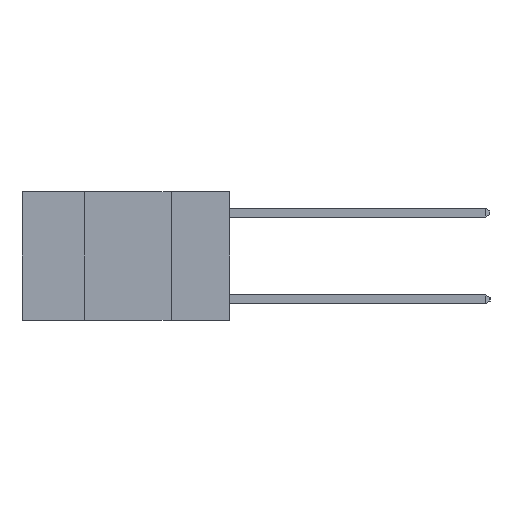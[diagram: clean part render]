
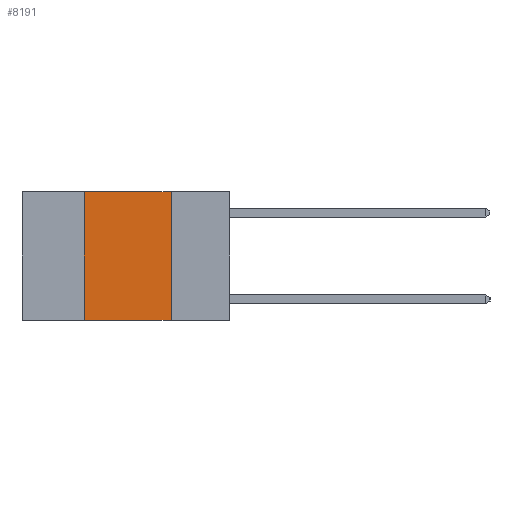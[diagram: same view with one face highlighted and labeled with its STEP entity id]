
A CAD part, left-side view. The second image highlights one B-rep face of the part: STEP entity #8191.
In plain terms, the highlighted planar face has unit normal (-1, 0, 0).
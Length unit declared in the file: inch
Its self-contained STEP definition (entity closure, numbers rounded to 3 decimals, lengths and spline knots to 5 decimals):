
#78 = CARTESIAN_POINT ( 'NONE',  ( 0., 0.42, 0. ) ) ;
#105 = ORIENTED_EDGE ( 'NONE', *, *, #7610, .F. ) ;
#230 = ORIENTED_EDGE ( 'NONE', *, *, #1454, .F. ) ;
#549 = CARTESIAN_POINT ( 'NONE',  ( 0., 0.17, -0.37 ) ) ;
#808 = VECTOR ( 'NONE', #7564, 39.37008 ) ;
#1454 = EDGE_CURVE ( 'NONE', #3037, #4385, #11405, .T. ) ;
#1978 = LINE ( 'NONE', #10693, #6566 ) ;
#1998 = EDGE_CURVE ( 'NONE', #4385, #9702, #5747, .T. ) ;
#2084 = CARTESIAN_POINT ( 'NONE',  ( 0., 0.6, 0. ) ) ;
#2086 = EDGE_CURVE ( 'NONE', #3037, #3465, #9427, .T. ) ;
#2439 = PLANE ( 'NONE',  #2926 ) ;
#2926 = AXIS2_PLACEMENT_3D ( 'NONE', #4290, #10646, #5195 ) ;
#3037 = VERTEX_POINT ( 'NONE', #10985 ) ;
#3465 = VERTEX_POINT ( 'NONE', #549 ) ;
#4176 = VECTOR ( 'NONE', #5009, 39.37008 ) ;
#4290 = CARTESIAN_POINT ( 'NONE',  ( 0., 0.6, 0. ) ) ;
#4385 = VERTEX_POINT ( 'NONE', #78 ) ;
#4529 = EDGE_LOOP ( 'NONE', ( #105, #7155, #230, #6249 ) ) ;
#5009 = DIRECTION ( 'NONE',  ( 0., 0., 1. ) ) ;
#5195 = DIRECTION ( 'NONE',  ( 0., 0., -1. ) ) ;
#5747 = LINE ( 'NONE', #2084, #808 ) ;
#6169 = DIRECTION ( 'NONE',  ( 0., 0., -1. ) ) ;
#6249 = ORIENTED_EDGE ( 'NONE', *, *, #2086, .T. ) ;
#6566 = VECTOR ( 'NONE', #6169, 39.37008 ) ;
#6991 = VECTOR ( 'NONE', #9535, 39.37008 ) ;
#7155 = ORIENTED_EDGE ( 'NONE', *, *, #1998, .F. ) ;
#7503 = CARTESIAN_POINT ( 'NONE',  ( 0., 0.17, 0. ) ) ;
#7564 = DIRECTION ( 'NONE',  ( 0., -1., 0. ) ) ;
#7610 = EDGE_CURVE ( 'NONE', #9702, #3465, #1978, .T. ) ;
#8191 = ADVANCED_FACE ( 'NONE', ( #8566 ), #2439, .F. ) ;
#8566 = FACE_OUTER_BOUND ( 'NONE', #4529, .T. ) ;
#8625 = CARTESIAN_POINT ( 'NONE',  ( 0., 0.6, -0.37 ) ) ;
#9427 = LINE ( 'NONE', #8625, #6991 ) ;
#9535 = DIRECTION ( 'NONE',  ( 0., -1., 0. ) ) ;
#9548 = CARTESIAN_POINT ( 'NONE',  ( 0., 0.42, 0. ) ) ;
#9702 = VERTEX_POINT ( 'NONE', #7503 ) ;
#10646 = DIRECTION ( 'NONE',  ( 1., 0., 0. ) ) ;
#10693 = CARTESIAN_POINT ( 'NONE',  ( 0., 0.17, 0. ) ) ;
#10985 = CARTESIAN_POINT ( 'NONE',  ( 0., 0.42, -0.37 ) ) ;
#11405 = LINE ( 'NONE', #9548, #4176 ) ;
